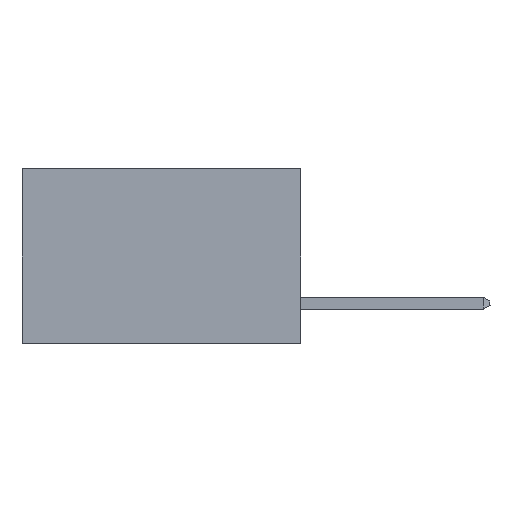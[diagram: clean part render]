
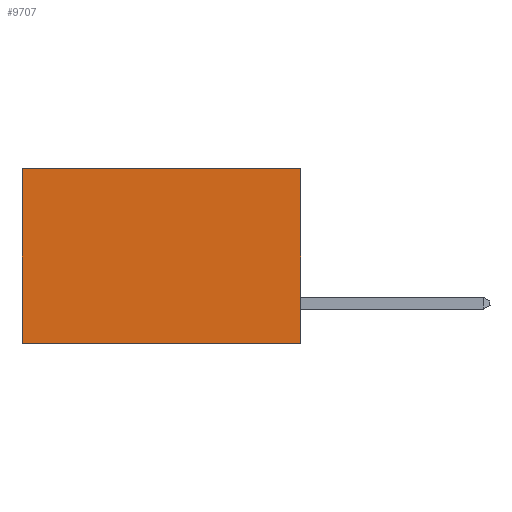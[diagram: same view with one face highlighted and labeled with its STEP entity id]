
A CAD part, left-side view. The second image highlights one B-rep face of the part: STEP entity #9707.
In plain terms, the highlighted planar face has unit normal (-1, 0, 0).
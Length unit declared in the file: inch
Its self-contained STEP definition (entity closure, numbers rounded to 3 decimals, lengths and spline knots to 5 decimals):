
#114 = ORIENTED_EDGE ( 'NONE', *, *, #9592, .T. ) ;
#356 = VECTOR ( 'NONE', #10693, 39.37008 ) ;
#702 = CARTESIAN_POINT ( 'NONE',  ( 0.277, 0., -0.37 ) ) ;
#1506 = EDGE_CURVE ( 'NONE', #15151, #12020, #17619, .T. ) ;
#1908 = DIRECTION ( 'NONE',  ( 1., 0., 0. ) ) ;
#2791 = LINE ( 'NONE', #702, #11973 ) ;
#2878 = CARTESIAN_POINT ( 'NONE',  ( 0.277, 0., 0. ) ) ;
#3658 = EDGE_CURVE ( 'NONE', #5094, #17668, #5623, .T. ) ;
#4388 = ORIENTED_EDGE ( 'NONE', *, *, #13463, .F. ) ;
#5094 = VERTEX_POINT ( 'NONE', #2878 ) ;
#5623 = LINE ( 'NONE', #14988, #18047 ) ;
#5905 = ORIENTED_EDGE ( 'NONE', *, *, #1506, .F. ) ;
#6018 = CARTESIAN_POINT ( 'NONE',  ( 0.277, 0.59, 0. ) ) ;
#6477 = CARTESIAN_POINT ( 'NONE',  ( 0.277, 0.59, -0.37 ) ) ;
#6679 = ORIENTED_EDGE ( 'NONE', *, *, #3658, .T. ) ;
#6883 = EDGE_LOOP ( 'NONE', ( #114, #5905, #4388, #6679 ) ) ;
#8471 = FACE_OUTER_BOUND ( 'NONE', #6883, .T. ) ;
#9592 = EDGE_CURVE ( 'NONE', #17668, #12020, #11011, .T. ) ;
#9707 = ADVANCED_FACE ( 'NONE', ( #8471 ), #10046, .F. ) ;
#10046 = PLANE ( 'NONE',  #10685 ) ;
#10685 = AXIS2_PLACEMENT_3D ( 'NONE', #11676, #1908, #13301 ) ;
#10693 = DIRECTION ( 'NONE',  ( 0., 1., 0. ) ) ;
#11011 = LINE ( 'NONE', #6477, #19102 ) ;
#11676 = CARTESIAN_POINT ( 'NONE',  ( 0.277, 0., -0.37 ) ) ;
#11973 = VECTOR ( 'NONE', #13755, 39.37008 ) ;
#12020 = VERTEX_POINT ( 'NONE', #13148 ) ;
#12943 = DIRECTION ( 'NONE',  ( 0., 0., -1. ) ) ;
#13148 = CARTESIAN_POINT ( 'NONE',  ( 0.277, 0.59, -0.37 ) ) ;
#13301 = DIRECTION ( 'NONE',  ( 0., 0., -1. ) ) ;
#13463 = EDGE_CURVE ( 'NONE', #5094, #15151, #2791, .T. ) ;
#13755 = DIRECTION ( 'NONE',  ( 0., 0., -1. ) ) ;
#13965 = CARTESIAN_POINT ( 'NONE',  ( 0.277, 0., -0.37 ) ) ;
#14108 = DIRECTION ( 'NONE',  ( 0., 1., 0. ) ) ;
#14988 = CARTESIAN_POINT ( 'NONE',  ( 0.277, 0., 0. ) ) ;
#15151 = VERTEX_POINT ( 'NONE', #13965 ) ;
#17619 = LINE ( 'NONE', #20480, #356 ) ;
#17668 = VERTEX_POINT ( 'NONE', #6018 ) ;
#18047 = VECTOR ( 'NONE', #14108, 39.37008 ) ;
#19102 = VECTOR ( 'NONE', #12943, 39.37008 ) ;
#20480 = CARTESIAN_POINT ( 'NONE',  ( 0.277, 0., -0.37 ) ) ;
